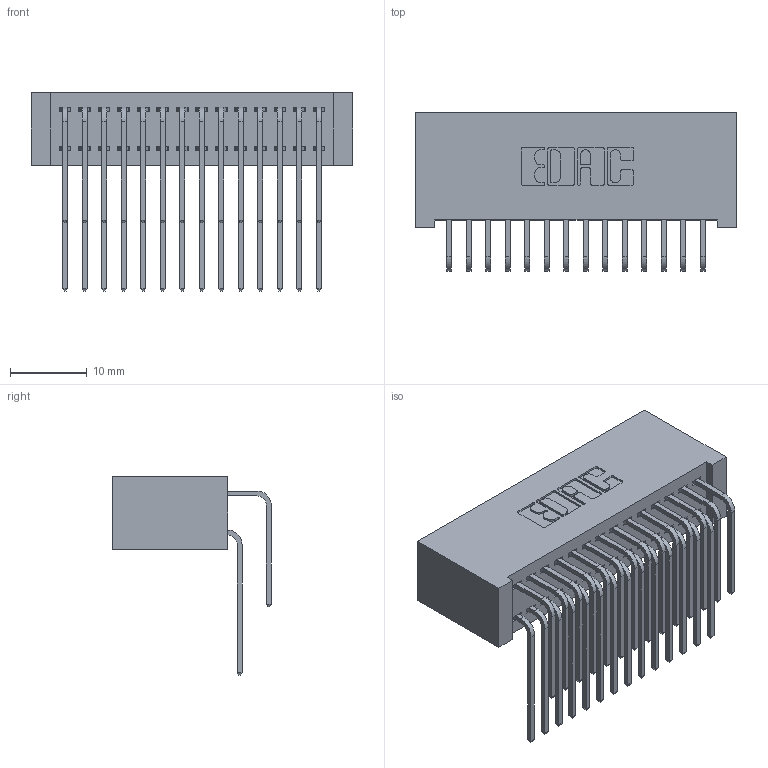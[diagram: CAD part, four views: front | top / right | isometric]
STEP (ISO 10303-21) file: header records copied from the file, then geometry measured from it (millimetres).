
FILE_DESCRIPTION (( 'STEP AP203' ), '1' );
FILE_NAME ('392-028-559-201.STEP', '2018-08-15T21:32:29', ( '' ), ( '' ), 'SwSTEP 2.0', 'SolidWorks 2016', '' );
FILE_SCHEMA (( 'CONFIG_CONTROL_DESIGN' ));
Length unit declared in the file: inch
Products named in the file (4): 342 Part_Lugless; 345-292-001_558 559 Tail - 1; 345-292-001_559 Tail - 2; 392-028-559-201
Assembly tree (29 placements, depth 2):
  392-028-559-201
    342 Part_Lugless
    345-292-001_558 559 Tail - 1  x14
    345-292-001_559 Tail - 2  x14
Bounding box: 41.81 x 20.64 x 25.78 mm (x, y, z)
Volume: 4225 mm3; surface area: 7364.2 mm2
Topology: 29 solids, 29 shells, 1614 faces, 4783 edges, 3150 vertices
Faces by surface type: plane 1126, cylinder 488
Entity records: 14003 total; most frequent: CARTESIAN_POINT 2401, ORIENTED_EDGE 2286, DIRECTION 2075, EDGE_CURVE 1143, LINE 983, VECTOR 983, VERTEX_POINT 758, AXIS2_PLACEMENT_3D 546
